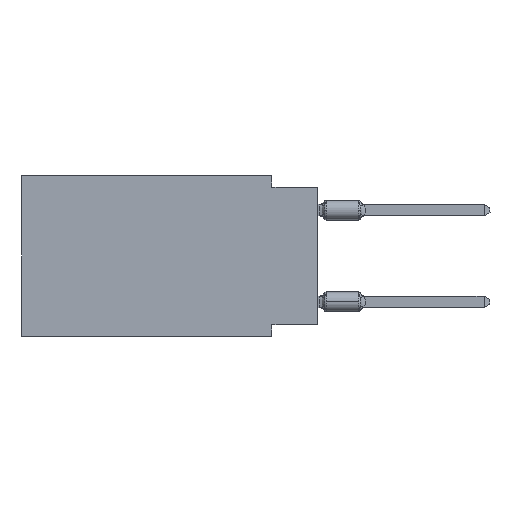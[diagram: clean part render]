
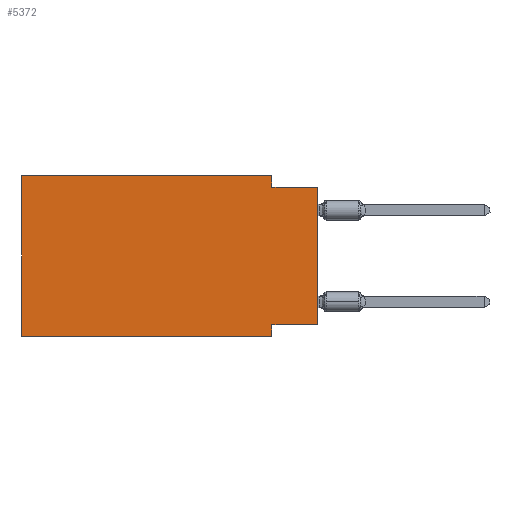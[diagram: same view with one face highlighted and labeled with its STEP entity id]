
A CAD part, left-side view. The second image highlights one B-rep face of the part: STEP entity #5372.
In plain terms, the highlighted planar face has unit normal (-1, 0, 0).
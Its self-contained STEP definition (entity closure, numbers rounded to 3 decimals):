
#279 = VECTOR ( 'NONE', #5511, 1000. ) ;
#1243 = VECTOR ( 'NONE', #3541, 1000. ) ;
#1453 = EDGE_CURVE ( 'NONE', #7251, #8355, #9440, .T. ) ;
#1948 = VERTEX_POINT ( 'NONE', #10313 ) ;
#2038 = CARTESIAN_POINT ( 'NONE',  ( 0., 0., -0.635 ) ) ;
#2165 = LINE ( 'NONE', #2038, #1243 ) ;
#2332 = CARTESIAN_POINT ( 'NONE',  ( 0., 2.54, -8.89 ) ) ;
#2384 = VERTEX_POINT ( 'NONE', #19936 ) ;
#2762 = LINE ( 'NONE', #22100, #18872 ) ;
#3337 = CARTESIAN_POINT ( 'NONE',  ( 0., 16.383, 0. ) ) ;
#3515 = VECTOR ( 'NONE', #19235, 1000. ) ;
#3541 = DIRECTION ( 'NONE',  ( 0., -1., 0. ) ) ;
#3609 = CARTESIAN_POINT ( 'NONE',  ( 0., 0., 0. ) ) ;
#4249 = ORIENTED_EDGE ( 'NONE', *, *, #11593, .F. ) ;
#4587 = DIRECTION ( 'NONE',  ( 0., 0., -1. ) ) ;
#5275 = LINE ( 'NONE', #10469, #19019 ) ;
#5372 = ADVANCED_FACE ( 'NONE', ( #14190 ), #17752, .F. ) ;
#5511 = DIRECTION ( 'NONE',  ( 0., 0., 1. ) ) ;
#5718 = VECTOR ( 'NONE', #17419, 1000. ) ;
#7251 = VERTEX_POINT ( 'NONE', #10493 ) ;
#7602 = CARTESIAN_POINT ( 'NONE',  ( 0., 16.383, -8.89 ) ) ;
#7801 = VECTOR ( 'NONE', #8628, 1000. ) ;
#8355 = VERTEX_POINT ( 'NONE', #2332 ) ;
#8571 = ORIENTED_EDGE ( 'NONE', *, *, #8855, .F. ) ;
#8608 = LINE ( 'NONE', #3337, #279 ) ;
#8628 = DIRECTION ( 'NONE',  ( 0., -1., 0. ) ) ;
#8855 = EDGE_CURVE ( 'NONE', #7251, #20595, #8608, .T. ) ;
#8891 = EDGE_CURVE ( 'NONE', #1948, #10850, #5275, .T. ) ;
#9440 = LINE ( 'NONE', #7602, #19355 ) ;
#9842 = EDGE_CURVE ( 'NONE', #22310, #21612, #2165, .T. ) ;
#10313 = CARTESIAN_POINT ( 'NONE',  ( 0., 0., -8.255 ) ) ;
#10427 = CARTESIAN_POINT ( 'NONE',  ( 0., 2.54, 0. ) ) ;
#10469 = CARTESIAN_POINT ( 'NONE',  ( 0., 0., -8.255 ) ) ;
#10493 = CARTESIAN_POINT ( 'NONE',  ( 0., 16.383, -8.89 ) ) ;
#10809 = DIRECTION ( 'NONE',  ( 0., 1., 0. ) ) ;
#10850 = VERTEX_POINT ( 'NONE', #21538 ) ;
#10872 = DIRECTION ( 'NONE',  ( 1., 0., 0. ) ) ;
#10992 = AXIS2_PLACEMENT_3D ( 'NONE', #15686, #10872, #22739 ) ;
#11593 = EDGE_CURVE ( 'NONE', #2384, #22310, #12593, .T. ) ;
#12471 = LINE ( 'NONE', #3609, #3515 ) ;
#12593 = LINE ( 'NONE', #10427, #5718 ) ;
#12791 = CARTESIAN_POINT ( 'NONE',  ( 0., 2.54, -0.635 ) ) ;
#12984 = CARTESIAN_POINT ( 'NONE',  ( 0., 0., -0.635 ) ) ;
#13342 = EDGE_CURVE ( 'NONE', #1948, #21612, #12471, .T. ) ;
#13912 = ORIENTED_EDGE ( 'NONE', *, *, #1453, .T. ) ;
#14072 = EDGE_LOOP ( 'NONE', ( #19250, #19018, #4249, #20565, #8571, #13912, #16960, #21401 ) ) ;
#14190 = FACE_OUTER_BOUND ( 'NONE', #14072, .T. ) ;
#15643 = CARTESIAN_POINT ( 'NONE',  ( 0., 16.383, 0. ) ) ;
#15686 = CARTESIAN_POINT ( 'NONE',  ( 0., 16.383, 0. ) ) ;
#15801 = EDGE_CURVE ( 'NONE', #20595, #2384, #19555, .T. ) ;
#16960 = ORIENTED_EDGE ( 'NONE', *, *, #17370, .F. ) ;
#17370 = EDGE_CURVE ( 'NONE', #10850, #8355, #2762, .T. ) ;
#17419 = DIRECTION ( 'NONE',  ( 0., 0., -1. ) ) ;
#17752 = PLANE ( 'NONE',  #10992 ) ;
#18872 = VECTOR ( 'NONE', #4587, 1000. ) ;
#19018 = ORIENTED_EDGE ( 'NONE', *, *, #9842, .F. ) ;
#19019 = VECTOR ( 'NONE', #10809, 1000. ) ;
#19235 = DIRECTION ( 'NONE',  ( 0., 0., 1. ) ) ;
#19250 = ORIENTED_EDGE ( 'NONE', *, *, #13342, .T. ) ;
#19355 = VECTOR ( 'NONE', #21414, 1000. ) ;
#19555 = LINE ( 'NONE', #15643, #7801 ) ;
#19936 = CARTESIAN_POINT ( 'NONE',  ( 0., 2.54, 0. ) ) ;
#20565 = ORIENTED_EDGE ( 'NONE', *, *, #15801, .F. ) ;
#20595 = VERTEX_POINT ( 'NONE', #22514 ) ;
#21401 = ORIENTED_EDGE ( 'NONE', *, *, #8891, .F. ) ;
#21414 = DIRECTION ( 'NONE',  ( 0., -1., 0. ) ) ;
#21538 = CARTESIAN_POINT ( 'NONE',  ( 0., 2.54, -8.255 ) ) ;
#21612 = VERTEX_POINT ( 'NONE', #12984 ) ;
#22100 = CARTESIAN_POINT ( 'NONE',  ( 0., 2.54, -8.89 ) ) ;
#22310 = VERTEX_POINT ( 'NONE', #12791 ) ;
#22514 = CARTESIAN_POINT ( 'NONE',  ( 0., 16.383, 0. ) ) ;
#22739 = DIRECTION ( 'NONE',  ( 0., 0., -1. ) ) ;
